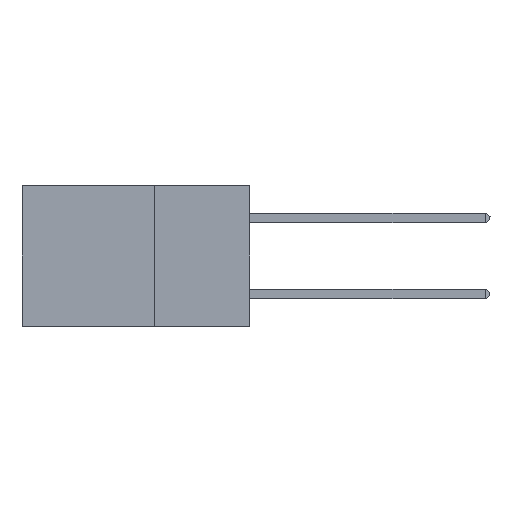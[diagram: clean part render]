
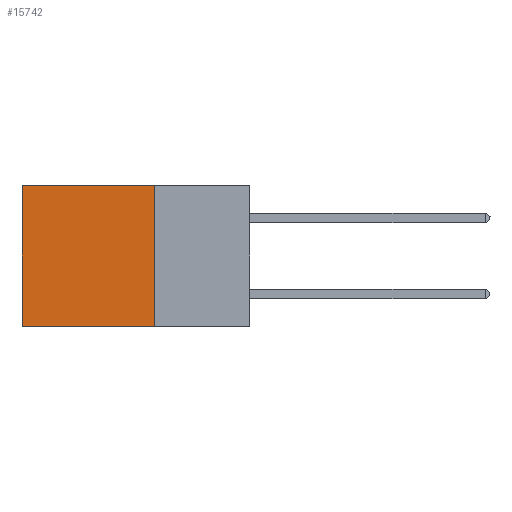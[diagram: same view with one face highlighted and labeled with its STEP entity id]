
A CAD part, left-side view. The second image highlights one B-rep face of the part: STEP entity #15742.
In plain terms, the highlighted planar face has unit normal (-1, 0, 0).
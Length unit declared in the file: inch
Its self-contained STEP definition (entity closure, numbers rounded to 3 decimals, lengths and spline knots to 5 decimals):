
#1000 = DIRECTION ( 'NONE',  ( 1., 0., 0. ) ) ;
#2632 = CARTESIAN_POINT ( 'NONE',  ( 0.2875, 0.6, -0.37 ) ) ;
#3056 = VECTOR ( 'NONE', #16894, 39.37008 ) ;
#4924 = VERTEX_POINT ( 'NONE', #19878 ) ;
#5352 = ORIENTED_EDGE ( 'NONE', *, *, #14339, .T. ) ;
#5669 = DIRECTION ( 'NONE',  ( 0., 0., -1. ) ) ;
#5670 = VERTEX_POINT ( 'NONE', #24737 ) ;
#5863 = PLANE ( 'NONE',  #15914 ) ;
#7165 = DIRECTION ( 'NONE',  ( 0., 0., -1. ) ) ;
#7198 = VERTEX_POINT ( 'NONE', #24629 ) ;
#8229 = LINE ( 'NONE', #15748, #14204 ) ;
#9617 = EDGE_CURVE ( 'NONE', #5670, #7198, #18257, .T. ) ;
#10507 = EDGE_CURVE ( 'NONE', #5670, #4924, #8229, .T. ) ;
#10887 = VECTOR ( 'NONE', #16758, 39.37008 ) ;
#11288 = ORIENTED_EDGE ( 'NONE', *, *, #10507, .F. ) ;
#11634 = EDGE_LOOP ( 'NONE', ( #5352, #20338, #11288, #20606 ) ) ;
#13701 = DIRECTION ( 'NONE',  ( 0., 0., -1. ) ) ;
#14204 = VECTOR ( 'NONE', #7165, 39.37008 ) ;
#14339 = EDGE_CURVE ( 'NONE', #7198, #16745, #19874, .T. ) ;
#15359 = EDGE_CURVE ( 'NONE', #4924, #16745, #20469, .T. ) ;
#15742 = ADVANCED_FACE ( 'NONE', ( #26054 ), #5863, .F. ) ;
#15748 = CARTESIAN_POINT ( 'NONE',  ( 0.2875, 0.25, 0. ) ) ;
#15914 = AXIS2_PLACEMENT_3D ( 'NONE', #26806, #1000, #13701 ) ;
#16092 = CARTESIAN_POINT ( 'NONE',  ( 0.2875, 0.6, 0. ) ) ;
#16745 = VERTEX_POINT ( 'NONE', #2632 ) ;
#16758 = DIRECTION ( 'NONE',  ( 0., 1., 0. ) ) ;
#16894 = DIRECTION ( 'NONE',  ( 0., 1., 0. ) ) ;
#18257 = LINE ( 'NONE', #23520, #3056 ) ;
#18901 = VECTOR ( 'NONE', #5669, 39.37008 ) ;
#19874 = LINE ( 'NONE', #16092, #18901 ) ;
#19878 = CARTESIAN_POINT ( 'NONE',  ( 0.2875, 0.25, -0.37 ) ) ;
#20338 = ORIENTED_EDGE ( 'NONE', *, *, #15359, .F. ) ;
#20469 = LINE ( 'NONE', #22735, #10887 ) ;
#20606 = ORIENTED_EDGE ( 'NONE', *, *, #9617, .T. ) ;
#22735 = CARTESIAN_POINT ( 'NONE',  ( 0.2875, 0.25, -0.37 ) ) ;
#23520 = CARTESIAN_POINT ( 'NONE',  ( 0.2875, 0.25, 0. ) ) ;
#24629 = CARTESIAN_POINT ( 'NONE',  ( 0.2875, 0.6, 0. ) ) ;
#24737 = CARTESIAN_POINT ( 'NONE',  ( 0.2875, 0.25, 0. ) ) ;
#26054 = FACE_OUTER_BOUND ( 'NONE', #11634, .T. ) ;
#26806 = CARTESIAN_POINT ( 'NONE',  ( 0.2875, 0.25, 0. ) ) ;
